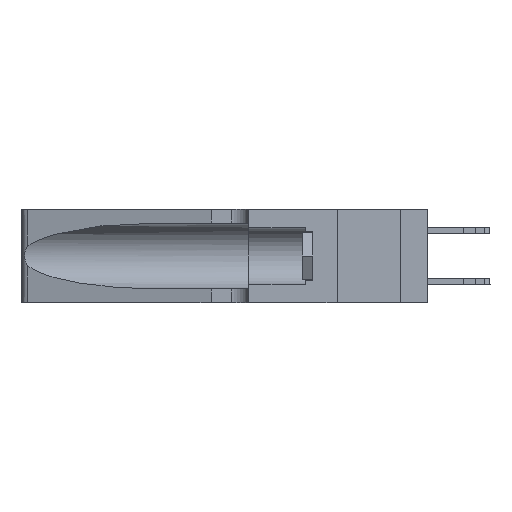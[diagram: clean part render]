
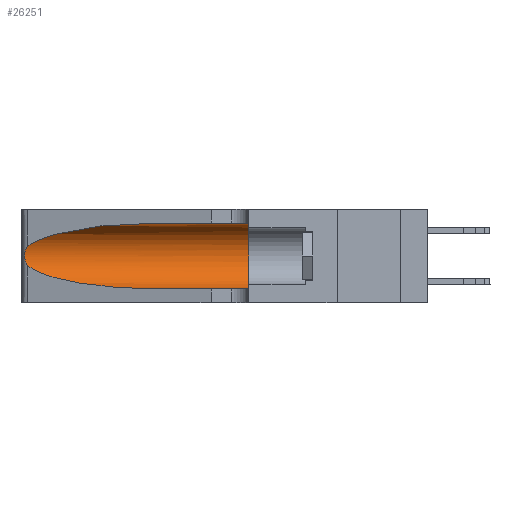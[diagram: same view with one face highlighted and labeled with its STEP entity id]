
A CAD part, left-side view. The second image highlights one B-rep face of the part: STEP entity #26251.
In plain terms, the highlighted cylindrical face has radius 3.308 mm (diameter 6.617 mm), a partial arc.
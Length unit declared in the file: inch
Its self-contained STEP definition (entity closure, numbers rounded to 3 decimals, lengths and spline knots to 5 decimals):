
#561 = CARTESIAN_POINT ( 'NONE',  ( 0.1305, 1.61858, 0.31525 ) ) ;
#695 = AXIS2_PLACEMENT_3D ( 'NONE', #2826, #28030, #15536 ) ;
#841 = EDGE_CURVE ( 'NONE', #27475, #14803, #28077, .T. ) ;
#1014 = EDGE_CURVE ( 'NONE', #28871, #28017, #28194, .T. ) ;
#1932 = ORIENTED_EDGE ( 'NONE', *, *, #1014, .F. ) ;
#2542 = EDGE_CURVE ( 'NONE', #14570, #27475, #22300, .T. ) ;
#2826 = CARTESIAN_POINT ( 'NONE',  ( 0.1305, 1.61858, 0.185 ) ) ;
#3041 = ORIENTED_EDGE ( 'NONE', *, *, #2542, .T. ) ;
#3115 = DIRECTION ( 'NONE',  ( 0., -1., 0. ) ) ;
#3323 = CARTESIAN_POINT ( 'NONE',  ( 0.2373, 1.15595, 0.28018 ) ) ;
#3440 = EDGE_LOOP ( 'NONE', ( #3945, #3041, #21270, #6586, #1932, #31286 ) ) ;
#3945 = ORIENTED_EDGE ( 'NONE', *, *, #17132, .T. ) ;
#5276 = CARTESIAN_POINT ( 'NONE',  ( 0.25854, 1.2359, 0.20912 ) ) ;
#6116 = LINE ( 'NONE', #21324, #22503 ) ;
#6586 = ORIENTED_EDGE ( 'NONE', *, *, #12211, .T. ) ;
#8047 = CARTESIAN_POINT ( 'NONE',  ( 0.26075, 1.23896, 0.19203 ) ) ;
#8217 = DIRECTION ( 'NONE',  ( 0., 0., 1. ) ) ;
#8344 = CARTESIAN_POINT ( 'NONE',  ( 0.18966, 0.96281, 0.31525 ) ) ;
#10391 = CARTESIAN_POINT ( 'NONE',  ( 0.1305, 0.35, 0.185 ) ) ;
#11060 = CARTESIAN_POINT ( 'NONE',  ( 0.25487, 1.22718, 0.22369 ) ) ;
#12211 = EDGE_CURVE ( 'NONE', #14803, #28017, #6116, .T. ) ;
#12599 = CYLINDRICAL_SURFACE ( 'NONE', #695, 0.13025 ) ;
#13102 = CARTESIAN_POINT ( 'NONE',  ( 0.25789, 1.23486, 0.15765 ) ) ;
#14570 = VERTEX_POINT ( 'NONE', #18903 ) ;
#14803 = VERTEX_POINT ( 'NONE', #24409 ) ;
#15186 = CARTESIAN_POINT ( 'NONE',  ( 0.25639, 1.23184, 0.21858 ) ) ;
#15536 = DIRECTION ( 'NONE',  ( 0., 0., -1. ) ) ;
#15909 = CARTESIAN_POINT ( 'NONE',  ( 0.1305, 0.72297, 0.31525 ) ) ;
#17132 = EDGE_CURVE ( 'NONE', #19509, #14570, #27274, .T. ) ;
#17838 = CARTESIAN_POINT ( 'NONE',  ( 0.25487, 1.22718, 0.14631 ) ) ;
#18239 = CARTESIAN_POINT ( 'NONE',  ( 0.1305, 0.72297, 0.31525 ) ) ;
#18482 = CARTESIAN_POINT ( 'NONE',  ( 0.25856, 1.23593, 0.16098 ) ) ;
#18633 = CARTESIAN_POINT ( 'NONE',  ( 0.25487, 1.22718, 0.22369 ) ) ;
#18903 = CARTESIAN_POINT ( 'NONE',  ( 0.25487, 1.22718, 0.22369 ) ) ;
#19509 = VERTEX_POINT ( 'NONE', #15909 ) ;
#20364 = CARTESIAN_POINT ( 'NONE',  ( 0.25787, 1.23484, 0.2124 ) ) ;
#20538 = CARTESIAN_POINT ( 'NONE',  ( 0.1305, 0.35, 0.31525 ) ) ;
#20674 = CARTESIAN_POINT ( 'NONE',  ( 0.25639, 1.23186, 0.15144 ) ) ;
#20789 = VECTOR ( 'NONE', #3115, 39.37008 ) ;
#21069 = DIRECTION ( 'NONE',  ( 0., 1., 0. ) ) ;
#21270 = ORIENTED_EDGE ( 'NONE', *, *, #841, .T. ) ;
#21324 = CARTESIAN_POINT ( 'NONE',  ( 0.1305, 1.61858, 0.05475 ) ) ;
#21439 = CARTESIAN_POINT ( 'NONE',  ( 0.25487, 1.22718, 0.14631 ) ) ;
#21594 = LINE ( 'NONE', #561, #20789 ) ;
#22300 = B_SPLINE_CURVE_WITH_KNOTS ( 'NONE', 3,
 ( #18633, #22679, #15186, #20364, #5276, #25402, #8047, #25609, #23325, #18482, #13102, #20674, #24086, #21439 ),
 .UNSPECIFIED., .F., .F.,
 ( 4, 2, 2, 2, 2, 2, 4 ),
 ( 0., 0.00027, 0.00053, 0.00107, 0.0016, 0.00187, 0.00214 ),
 .UNSPECIFIED. ) ;
#22503 = VECTOR ( 'NONE', #30612, 39.37008 ) ;
#22679 = CARTESIAN_POINT ( 'NONE',  ( 0.25555, 1.22994, 0.2215 ) ) ;
#22714 = CARTESIAN_POINT ( 'NONE',  ( 0.1305, 0.35, 0.05475 ) ) ;
#23325 = CARTESIAN_POINT ( 'NONE',  ( 0.26017, 1.23833, 0.17102 ) ) ;
#24086 = CARTESIAN_POINT ( 'NONE',  ( 0.25555, 1.22993, 0.14849 ) ) ;
#24409 = CARTESIAN_POINT ( 'NONE',  ( 0.1305, 0.72297, 0.05475 ) ) ;
#24417 = FACE_OUTER_BOUND ( 'NONE', #3440, .T. ) ;
#24970 = CARTESIAN_POINT ( 'NONE',  ( 0.18966, 0.96281, 0.05475 ) ) ;
#25077 = CARTESIAN_POINT ( 'NONE',  ( 0.2373, 1.15595, 0.08982 ) ) ;
#25185 = CARTESIAN_POINT ( 'NONE',  ( 0.1305, 0.72297, 0.05475 ) ) ;
#25402 = CARTESIAN_POINT ( 'NONE',  ( 0.26018, 1.23835, 0.19895 ) ) ;
#25609 = CARTESIAN_POINT ( 'NONE',  ( 0.26075, 1.23896, 0.178 ) ) ;
#25875 = CARTESIAN_POINT ( 'NONE',  ( 0.25487, 1.22718, 0.14631 ) ) ;
#26251 = ADVANCED_FACE ( 'NONE', ( #24417 ), #12599, .F. ) ;
#26958 = EDGE_CURVE ( 'NONE', #19509, #28871, #21594, .T. ) ;
#27274 =( BOUNDED_CURVE ( )  B_SPLINE_CURVE ( 3, ( #18239, #8344, #3323, #11060 ),
 .UNSPECIFIED., .F., .F. ) 
 B_SPLINE_CURVE_WITH_KNOTS ( ( 4, 4 ),
 ( 1.5708, 2.84003 ),
 .UNSPECIFIED. ) 
 CURVE ( )  GEOMETRIC_REPRESENTATION_ITEM ( )  RATIONAL_B_SPLINE_CURVE ( ( 1., 0.87, 0.87, 1. ) ) 
 REPRESENTATION_ITEM ( '' )  );
#27475 = VERTEX_POINT ( 'NONE', #25875 ) ;
#28017 = VERTEX_POINT ( 'NONE', #22714 ) ;
#28030 = DIRECTION ( 'NONE',  ( 0., -1., 0. ) ) ;
#28077 =( BOUNDED_CURVE ( )  B_SPLINE_CURVE ( 3, ( #17838, #25077, #24970, #25185 ),
 .UNSPECIFIED., .F., .T. ) 
 B_SPLINE_CURVE_WITH_KNOTS ( ( 4, 4 ),
 ( 3.44316, 4.71239 ),
 .UNSPECIFIED. ) 
 CURVE ( )  GEOMETRIC_REPRESENTATION_ITEM ( )  RATIONAL_B_SPLINE_CURVE ( ( 1., 0.87, 0.87, 1. ) ) 
 REPRESENTATION_ITEM ( '' )  );
#28194 = CIRCLE ( 'NONE', #32159, 0.13025 ) ;
#28871 = VERTEX_POINT ( 'NONE', #20538 ) ;
#30612 = DIRECTION ( 'NONE',  ( 0., -1., 0. ) ) ;
#31286 = ORIENTED_EDGE ( 'NONE', *, *, #26958, .F. ) ;
#32159 = AXIS2_PLACEMENT_3D ( 'NONE', #10391, #21069, #8217 ) ;
